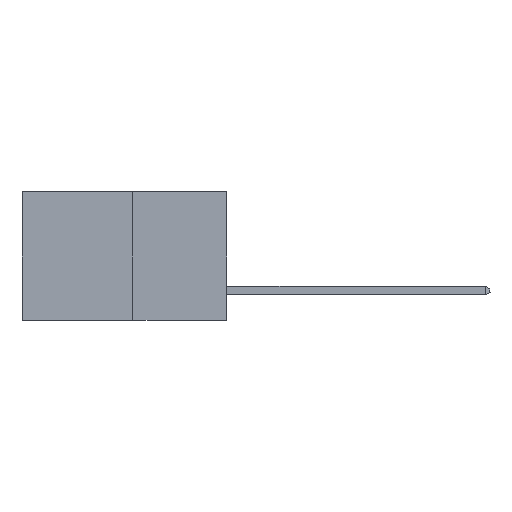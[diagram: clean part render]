
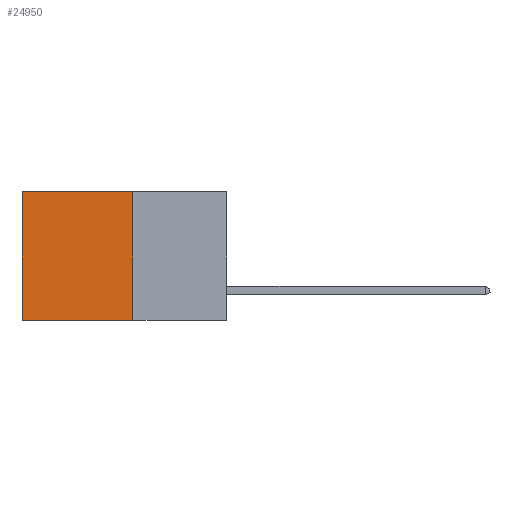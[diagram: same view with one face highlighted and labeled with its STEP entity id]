
A CAD part, left-side view. The second image highlights one B-rep face of the part: STEP entity #24950.
In plain terms, the highlighted planar face has unit normal (-1, 0, 0).
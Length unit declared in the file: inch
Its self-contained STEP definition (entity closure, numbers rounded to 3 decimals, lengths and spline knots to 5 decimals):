
#186 = AXIS2_PLACEMENT_3D ( 'NONE', #22000, #15865, #3256 ) ;
#1110 = PLANE ( 'NONE',  #186 ) ;
#1170 = VERTEX_POINT ( 'NONE', #24197 ) ;
#1651 = DIRECTION ( 'NONE',  ( 0., 1., 0. ) ) ;
#1952 = VECTOR ( 'NONE', #1651, 39.37008 ) ;
#2081 = ORIENTED_EDGE ( 'NONE', *, *, #11549, .F. ) ;
#2192 = VECTOR ( 'NONE', #21075, 39.37008 ) ;
#3256 = DIRECTION ( 'NONE',  ( 0., 0., -1. ) ) ;
#4842 = EDGE_CURVE ( 'NONE', #6302, #12661, #17952, .T. ) ;
#6180 = VECTOR ( 'NONE', #13965, 39.37008 ) ;
#6302 = VERTEX_POINT ( 'NONE', #8068 ) ;
#6511 = CARTESIAN_POINT ( 'NONE',  ( 0.277, 0.59, -0.37 ) ) ;
#6685 = CARTESIAN_POINT ( 'NONE',  ( 0.277, 0.59, -0.37 ) ) ;
#7493 = CARTESIAN_POINT ( 'NONE',  ( 0.277, 0.27, -0.37 ) ) ;
#8068 = CARTESIAN_POINT ( 'NONE',  ( 0.277, 0.27, 0. ) ) ;
#8311 = LINE ( 'NONE', #12193, #1952 ) ;
#9682 = FACE_OUTER_BOUND ( 'NONE', #10439, .T. ) ;
#10439 = EDGE_LOOP ( 'NONE', ( #18655, #2081, #22741, #12446 ) ) ;
#11549 = EDGE_CURVE ( 'NONE', #12661, #23330, #8311, .T. ) ;
#11846 = CARTESIAN_POINT ( 'NONE',  ( 0.277, 0.27, -0.37 ) ) ;
#12031 = CARTESIAN_POINT ( 'NONE',  ( 0.277, 0.27, 0. ) ) ;
#12193 = CARTESIAN_POINT ( 'NONE',  ( 0.277, 0.27, -0.37 ) ) ;
#12446 = ORIENTED_EDGE ( 'NONE', *, *, #18377, .T. ) ;
#12661 = VERTEX_POINT ( 'NONE', #7493 ) ;
#13965 = DIRECTION ( 'NONE',  ( 0., 0., -1. ) ) ;
#13998 = LINE ( 'NONE', #12031, #18880 ) ;
#15865 = DIRECTION ( 'NONE',  ( 1., 0., 0. ) ) ;
#16177 = DIRECTION ( 'NONE',  ( 0., 1., 0. ) ) ;
#17952 = LINE ( 'NONE', #11846, #6180 ) ;
#18377 = EDGE_CURVE ( 'NONE', #6302, #1170, #13998, .T. ) ;
#18655 = ORIENTED_EDGE ( 'NONE', *, *, #21435, .T. ) ;
#18880 = VECTOR ( 'NONE', #16177, 39.37008 ) ;
#21075 = DIRECTION ( 'NONE',  ( 0., 0., -1. ) ) ;
#21435 = EDGE_CURVE ( 'NONE', #1170, #23330, #23149, .T. ) ;
#22000 = CARTESIAN_POINT ( 'NONE',  ( 0.277, 0.27, -0.37 ) ) ;
#22741 = ORIENTED_EDGE ( 'NONE', *, *, #4842, .F. ) ;
#23149 = LINE ( 'NONE', #6511, #2192 ) ;
#23330 = VERTEX_POINT ( 'NONE', #6685 ) ;
#24197 = CARTESIAN_POINT ( 'NONE',  ( 0.277, 0.59, 0. ) ) ;
#24950 = ADVANCED_FACE ( 'NONE', ( #9682 ), #1110, .F. ) ;
